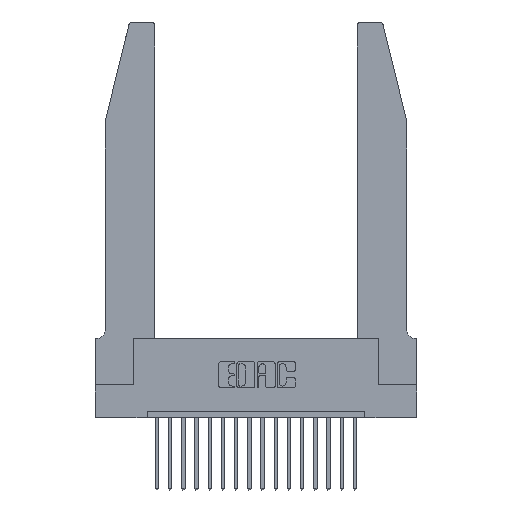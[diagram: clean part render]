
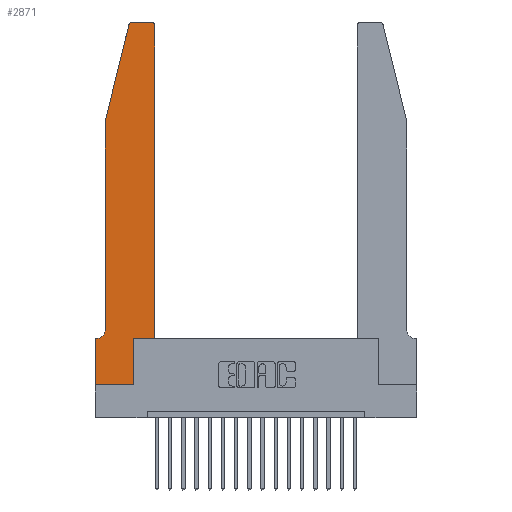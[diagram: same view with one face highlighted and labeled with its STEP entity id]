
A CAD part, top view. The second image highlights one B-rep face of the part: STEP entity #2871.
In plain terms, the highlighted planar face has unit normal (0, 0, 1).
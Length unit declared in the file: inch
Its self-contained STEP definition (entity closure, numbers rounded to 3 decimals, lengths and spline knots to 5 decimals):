
#145 = DIRECTION ( 'NONE',  ( 0., -1., 0. ) ) ;
#510 = EDGE_LOOP ( 'NONE', ( #18460, #14906, #4660, #3957, #9531, #15881, #10567, #7636, #8142, #4816, #11915, #16867 ) ) ;
#548 = EDGE_CURVE ( 'NONE', #773, #990, #14438, .T. ) ;
#773 = VERTEX_POINT ( 'NONE', #17659 ) ;
#805 = LINE ( 'NONE', #4024, #2782 ) ;
#990 = VERTEX_POINT ( 'NONE', #4268 ) ;
#1181 = CARTESIAN_POINT ( 'NONE',  ( 0.0055, 0.42, 0.37 ) ) ;
#1278 = EDGE_CURVE ( 'NONE', #8152, #8889, #15137, .T. ) ;
#1361 = AXIS2_PLACEMENT_3D ( 'NONE', #1181, #1396, #13739 ) ;
#1396 = DIRECTION ( 'NONE',  ( 0., 0., -1. ) ) ;
#1432 = DIRECTION ( 'NONE',  ( 0., 0., 1. ) ) ;
#1518 = CARTESIAN_POINT ( 'NONE',  ( 0.25487, 2.72718, 0.37 ) ) ;
#2027 = VECTOR ( 'NONE', #11651, 39.37008 ) ;
#2541 = VERTEX_POINT ( 'NONE', #11833 ) ;
#2597 = CARTESIAN_POINT ( 'NONE',  ( 0.0755, 2., 0.37 ) ) ;
#2782 = VECTOR ( 'NONE', #14732, 39.37008 ) ;
#2806 = CARTESIAN_POINT ( 'NONE',  ( 0.4205, 2.72, 0.37 ) ) ;
#2871 = ADVANCED_FACE ( 'NONE', ( #15583 ), #11372, .T. ) ;
#3412 = LINE ( 'NONE', #14672, #10530 ) ;
#3613 = CARTESIAN_POINT ( 'NONE',  ( 0.4505, 0.35, 0.37 ) ) ;
#3957 = ORIENTED_EDGE ( 'NONE', *, *, #12293, .T. ) ;
#4024 = CARTESIAN_POINT ( 'NONE',  ( 0., 0., 0.37 ) ) ;
#4268 = CARTESIAN_POINT ( 'NONE',  ( 0.4505, 0.35, 0.37 ) ) ;
#4372 = DIRECTION ( 'NONE',  ( 0., 0., 1. ) ) ;
#4660 = ORIENTED_EDGE ( 'NONE', *, *, #1278, .T. ) ;
#4697 = AXIS2_PLACEMENT_3D ( 'NONE', #14050, #1432, #7687 ) ;
#4751 = LINE ( 'NONE', #12511, #16759 ) ;
#4816 = ORIENTED_EDGE ( 'NONE', *, *, #548, .T. ) ;
#4936 = VERTEX_POINT ( 'NONE', #11194 ) ;
#5437 = VERTEX_POINT ( 'NONE', #7724 ) ;
#5609 = VECTOR ( 'NONE', #14834, 39.37008 ) ;
#6190 = CARTESIAN_POINT ( 'NONE',  ( 0.0755, 0.35, 0.37 ) ) ;
#6397 = VERTEX_POINT ( 'NONE', #7549 ) ;
#6949 = DIRECTION ( 'NONE',  ( 0., 1., 0. ) ) ;
#7549 = CARTESIAN_POINT ( 'NONE',  ( 0., 0.35, 0.37 ) ) ;
#7636 = ORIENTED_EDGE ( 'NONE', *, *, #19450, .T. ) ;
#7687 = DIRECTION ( 'NONE',  ( 1., 0., 0. ) ) ;
#7691 = CARTESIAN_POINT ( 'NONE',  ( 0.0755, 2., 0.37 ) ) ;
#7724 = CARTESIAN_POINT ( 'NONE',  ( 0.4505, 2.72, 0.37 ) ) ;
#8010 = EDGE_CURVE ( 'NONE', #9226, #6397, #14333, .T. ) ;
#8142 = ORIENTED_EDGE ( 'NONE', *, *, #10042, .T. ) ;
#8152 = VERTEX_POINT ( 'NONE', #1518 ) ;
#8414 = DIRECTION ( 'NONE',  ( 1., 0., 0. ) ) ;
#8889 = VERTEX_POINT ( 'NONE', #2597 ) ;
#9031 = CARTESIAN_POINT ( 'NONE',  ( 0.2605, 2.75, 0.37 ) ) ;
#9226 = VERTEX_POINT ( 'NONE', #19244 ) ;
#9531 = ORIENTED_EDGE ( 'NONE', *, *, #18545, .T. ) ;
#10022 = CARTESIAN_POINT ( 'NONE',  ( 0.4505, 0.35, 0.37 ) ) ;
#10042 = EDGE_CURVE ( 'NONE', #4936, #773, #14507, .T. ) ;
#10530 = VECTOR ( 'NONE', #13218, 39.37008 ) ;
#10538 = AXIS2_PLACEMENT_3D ( 'NONE', #2806, #4372, #12814 ) ;
#10567 = ORIENTED_EDGE ( 'NONE', *, *, #11808, .T. ) ;
#11194 = CARTESIAN_POINT ( 'NONE',  ( 0.2865, 0., 0.37 ) ) ;
#11288 = EDGE_CURVE ( 'NONE', #12025, #8152, #18368, .T. ) ;
#11372 = PLANE ( 'NONE',  #16417 ) ;
#11471 = LINE ( 'NONE', #9031, #19286 ) ;
#11651 = DIRECTION ( 'NONE',  ( 0., 1., 0. ) ) ;
#11699 = DIRECTION ( 'NONE',  ( 0., 0., 1. ) ) ;
#11808 = EDGE_CURVE ( 'NONE', #6397, #15775, #3412, .T. ) ;
#11833 = CARTESIAN_POINT ( 'NONE',  ( 0.4205, 2.75, 0.37 ) ) ;
#11861 = VERTEX_POINT ( 'NONE', #15789 ) ;
#11915 = ORIENTED_EDGE ( 'NONE', *, *, #18333, .T. ) ;
#12025 = VERTEX_POINT ( 'NONE', #16803 ) ;
#12293 = EDGE_CURVE ( 'NONE', #8889, #11861, #4751, .T. ) ;
#12416 = DIRECTION ( 'NONE',  ( -1., 0., 0. ) ) ;
#12511 = CARTESIAN_POINT ( 'NONE',  ( 0.0755, 2., 0.37 ) ) ;
#12555 = CARTESIAN_POINT ( 'NONE',  ( 0.2865, 0.35, 0.37 ) ) ;
#12814 = DIRECTION ( 'NONE',  ( 1., 0., 0. ) ) ;
#12913 = CARTESIAN_POINT ( 'NONE',  ( 0., 0.35, 0.37 ) ) ;
#12923 = VECTOR ( 'NONE', #18768, 39.37008 ) ;
#13218 = DIRECTION ( 'NONE',  ( 0., -1., 0. ) ) ;
#13739 = DIRECTION ( 'NONE',  ( -1., 0., 0. ) ) ;
#14050 = CARTESIAN_POINT ( 'NONE',  ( 0.284, 2.72, 0.37 ) ) ;
#14333 = LINE ( 'NONE', #6190, #20203 ) ;
#14438 = LINE ( 'NONE', #3613, #5609 ) ;
#14507 = LINE ( 'NONE', #12555, #20140 ) ;
#14672 = CARTESIAN_POINT ( 'NONE',  ( 0., 0., 0.37 ) ) ;
#14732 = DIRECTION ( 'NONE',  ( 1., 0., 0. ) ) ;
#14834 = DIRECTION ( 'NONE',  ( 1., 0., 0. ) ) ;
#14906 = ORIENTED_EDGE ( 'NONE', *, *, #11288, .T. ) ;
#15137 = LINE ( 'NONE', #7691, #12923 ) ;
#15583 = FACE_OUTER_BOUND ( 'NONE', #510, .T. ) ;
#15680 = DIRECTION ( 'NONE',  ( -1., 0., 0. ) ) ;
#15697 = EDGE_CURVE ( 'NONE', #2541, #12025, #11471, .T. ) ;
#15775 = VERTEX_POINT ( 'NONE', #20314 ) ;
#15789 = CARTESIAN_POINT ( 'NONE',  ( 0.0755, 0.42, 0.37 ) ) ;
#15881 = ORIENTED_EDGE ( 'NONE', *, *, #8010, .T. ) ;
#16417 = AXIS2_PLACEMENT_3D ( 'NONE', #12913, #11699, #8414 ) ;
#16759 = VECTOR ( 'NONE', #145, 39.37008 ) ;
#16803 = CARTESIAN_POINT ( 'NONE',  ( 0.284, 2.75, 0.37 ) ) ;
#16867 = ORIENTED_EDGE ( 'NONE', *, *, #17399, .T. ) ;
#17011 = CIRCLE ( 'NONE', #10538, 0.03 ) ;
#17399 = EDGE_CURVE ( 'NONE', #5437, #2541, #17011, .T. ) ;
#17659 = CARTESIAN_POINT ( 'NONE',  ( 0.2865, 0.35, 0.37 ) ) ;
#17709 = CIRCLE ( 'NONE', #1361, 0.07 ) ;
#18333 = EDGE_CURVE ( 'NONE', #990, #5437, #18704, .T. ) ;
#18368 = CIRCLE ( 'NONE', #4697, 0.03 ) ;
#18460 = ORIENTED_EDGE ( 'NONE', *, *, #15697, .T. ) ;
#18545 = EDGE_CURVE ( 'NONE', #11861, #9226, #17709, .T. ) ;
#18704 = LINE ( 'NONE', #10022, #2027 ) ;
#18768 = DIRECTION ( 'NONE',  ( -0.239, -0.971, 0. ) ) ;
#19244 = CARTESIAN_POINT ( 'NONE',  ( 0.0055, 0.35, 0.37 ) ) ;
#19286 = VECTOR ( 'NONE', #15680, 39.37008 ) ;
#19450 = EDGE_CURVE ( 'NONE', #15775, #4936, #805, .T. ) ;
#20140 = VECTOR ( 'NONE', #6949, 39.37008 ) ;
#20203 = VECTOR ( 'NONE', #12416, 39.37008 ) ;
#20314 = CARTESIAN_POINT ( 'NONE',  ( 0., 0., 0.37 ) ) ;
